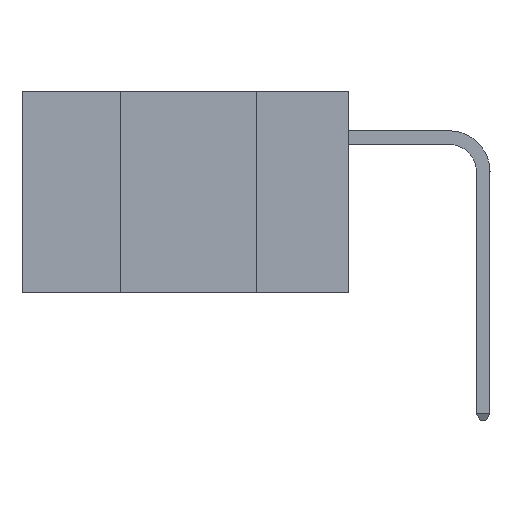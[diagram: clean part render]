
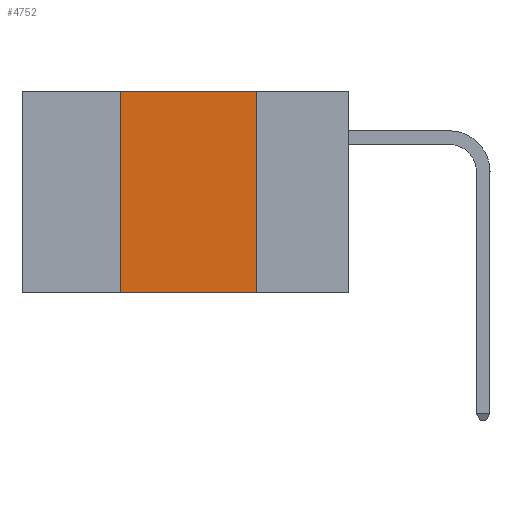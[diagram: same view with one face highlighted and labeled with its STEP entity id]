
A CAD part, left-side view. The second image highlights one B-rep face of the part: STEP entity #4752.
In plain terms, the highlighted planar face has unit normal (-1, 0, 0).
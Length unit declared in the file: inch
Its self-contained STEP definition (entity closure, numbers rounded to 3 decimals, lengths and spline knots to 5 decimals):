
#271 = ORIENTED_EDGE ( 'NONE', *, *, #1007, .F. ) ;
#839 = CARTESIAN_POINT ( 'NONE',  ( 0., 0.17, 0. ) ) ;
#1007 = EDGE_CURVE ( 'NONE', #44053, #19548, #18082, .T. ) ;
#3597 = CARTESIAN_POINT ( 'NONE',  ( 0., 0.6, 0. ) ) ;
#4439 = DIRECTION ( 'NONE',  ( 0., 0., -1. ) ) ;
#4752 = ADVANCED_FACE ( 'NONE', ( #11829 ), #18940, .F. ) ;
#8602 = VECTOR ( 'NONE', #21925, 39.37008 ) ;
#10722 = EDGE_CURVE ( 'NONE', #44053, #22697, #42735, .T. ) ;
#11829 = FACE_OUTER_BOUND ( 'NONE', #12166, .T. ) ;
#12025 = VECTOR ( 'NONE', #35425, 39.37008 ) ;
#12166 = EDGE_LOOP ( 'NONE', ( #43092, #28772, #271, #35468 ) ) ;
#15731 = EDGE_CURVE ( 'NONE', #38700, #22697, #27398, .T. ) ;
#18082 = LINE ( 'NONE', #23429, #8602 ) ;
#18940 = PLANE ( 'NONE',  #24051 ) ;
#19548 = VERTEX_POINT ( 'NONE', #32043 ) ;
#21925 = DIRECTION ( 'NONE',  ( 0., 0., 1. ) ) ;
#22584 = DIRECTION ( 'NONE',  ( 0., 0., -1. ) ) ;
#22697 = VERTEX_POINT ( 'NONE', #43057 ) ;
#23429 = CARTESIAN_POINT ( 'NONE',  ( 0., 0.42, 0. ) ) ;
#23908 = CARTESIAN_POINT ( 'NONE',  ( 0., 0.17, 0. ) ) ;
#24051 = AXIS2_PLACEMENT_3D ( 'NONE', #36779, #43830, #22584 ) ;
#27398 = LINE ( 'NONE', #839, #45011 ) ;
#27895 = CARTESIAN_POINT ( 'NONE',  ( 0., 0.6, -0.37 ) ) ;
#28772 = ORIENTED_EDGE ( 'NONE', *, *, #32219, .F. ) ;
#32043 = CARTESIAN_POINT ( 'NONE',  ( 0., 0.42, 0. ) ) ;
#32219 = EDGE_CURVE ( 'NONE', #19548, #38700, #39420, .T. ) ;
#34483 = VECTOR ( 'NONE', #38410, 39.37008 ) ;
#35425 = DIRECTION ( 'NONE',  ( 0., -1., 0. ) ) ;
#35468 = ORIENTED_EDGE ( 'NONE', *, *, #10722, .T. ) ;
#36779 = CARTESIAN_POINT ( 'NONE',  ( 0., 0.6, 0. ) ) ;
#38410 = DIRECTION ( 'NONE',  ( 0., -1., 0. ) ) ;
#38700 = VERTEX_POINT ( 'NONE', #23908 ) ;
#39420 = LINE ( 'NONE', #3597, #12025 ) ;
#39672 = CARTESIAN_POINT ( 'NONE',  ( 0., 0.42, -0.37 ) ) ;
#42735 = LINE ( 'NONE', #27895, #34483 ) ;
#43057 = CARTESIAN_POINT ( 'NONE',  ( 0., 0.17, -0.37 ) ) ;
#43092 = ORIENTED_EDGE ( 'NONE', *, *, #15731, .F. ) ;
#43830 = DIRECTION ( 'NONE',  ( 1., 0., 0. ) ) ;
#44053 = VERTEX_POINT ( 'NONE', #39672 ) ;
#45011 = VECTOR ( 'NONE', #4439, 39.37008 ) ;
